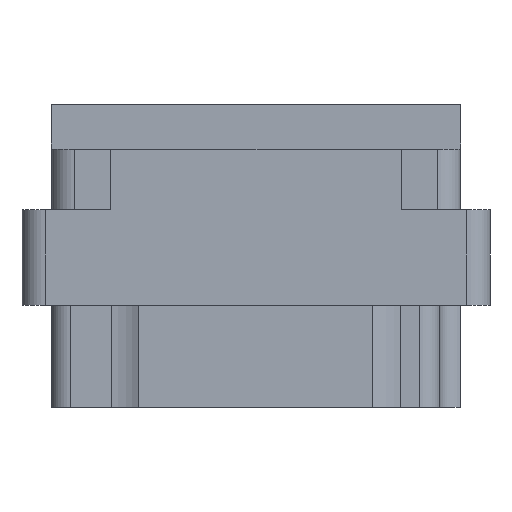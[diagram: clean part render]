
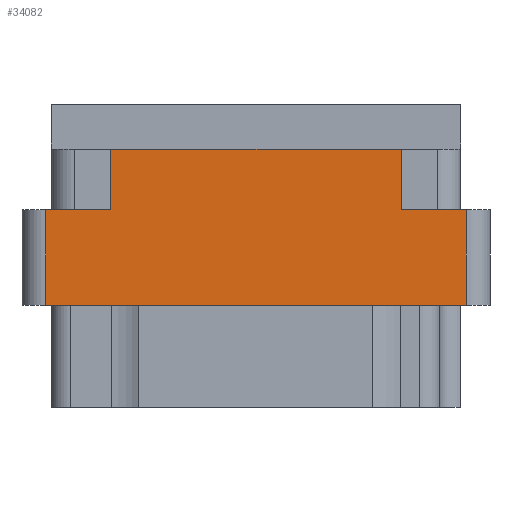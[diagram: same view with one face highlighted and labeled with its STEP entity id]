
A CAD part, left-side view. The second image highlights one B-rep face of the part: STEP entity #34082.
In plain terms, the highlighted planar face has unit normal (-1, 0, 0).
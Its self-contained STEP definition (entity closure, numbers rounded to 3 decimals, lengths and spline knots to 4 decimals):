
#12 = CARTESIAN_POINT ( 'NONE',  ( -1.359, 0.617, -0.117 ) ) ;
#473 = VECTOR ( 'NONE', #33977, 39.3701 ) ;
#823 = VERTEX_POINT ( 'NONE', #48554 ) ;
#3476 = EDGE_CURVE ( 'NONE', #823, #56466, #4564, .T. ) ;
#3737 = CARTESIAN_POINT ( 'NONE',  ( -1.359, -0.3825, -0.277 ) ) ;
#4472 = CARTESIAN_POINT ( 'NONE',  ( -1.359, -0.3825, -0.117 ) ) ;
#4564 = LINE ( 'NONE', #55939, #473 ) ;
#5445 = VERTEX_POINT ( 'NONE', #45463 ) ;
#5642 = VERTEX_POINT ( 'NONE', #42252 ) ;
#6634 = DIRECTION ( 'NONE',  ( 0., 0., 1. ) ) ;
#6751 = LINE ( 'NONE', #41311, #39908 ) ;
#8000 = LINE ( 'NONE', #8088, #42814 ) ;
#8088 = CARTESIAN_POINT ( 'NONE',  ( -1.359, 0.555, -0.798 ) ) ;
#11382 = VERTEX_POINT ( 'NONE', #18993 ) ;
#11663 = LINE ( 'NONE', #57375, #38190 ) ;
#14335 = LINE ( 'NONE', #16645, #18534 ) ;
#14770 = ORIENTED_EDGE ( 'NONE', *, *, #55445, .F. ) ;
#15271 = DIRECTION ( 'NONE',  ( 0., -1., 0. ) ) ;
#15533 = EDGE_CURVE ( 'NONE', #11382, #64321, #14335, .T. ) ;
#16645 = CARTESIAN_POINT ( 'NONE',  ( -1.359, 0., -0.529 ) ) ;
#18534 = VECTOR ( 'NONE', #21676, 39.3701 ) ;
#18692 = VERTEX_POINT ( 'NONE', #60002 ) ;
#18993 = CARTESIAN_POINT ( 'NONE',  ( -1.359, -0.555, -0.529 ) ) ;
#19235 = ORIENTED_EDGE ( 'NONE', *, *, #15533, .F. ) ;
#19709 = LINE ( 'NONE', #12, #23008 ) ;
#20293 = FACE_OUTER_BOUND ( 'NONE', #48943, .T. ) ;
#20583 = DIRECTION ( 'NONE',  ( 0., 0., 1. ) ) ;
#21238 = CARTESIAN_POINT ( 'NONE',  ( -1.359, 0.3825, -0.277 ) ) ;
#21350 = ORIENTED_EDGE ( 'NONE', *, *, #66584, .T. ) ;
#21676 = DIRECTION ( 'NONE',  ( 0., 1., 0. ) ) ;
#22832 = PLANE ( 'NONE',  #50138 ) ;
#23008 = VECTOR ( 'NONE', #15271, 39.3701 ) ;
#24571 = DIRECTION ( 'NONE',  ( 0., 0., 1. ) ) ;
#28092 = VECTOR ( 'NONE', #39802, 39.3701 ) ;
#28145 = EDGE_CURVE ( 'NONE', #11382, #5445, #11663, .T. ) ;
#29629 = CARTESIAN_POINT ( 'NONE',  ( -1.359, 0.3825, -0.277 ) ) ;
#30195 = ORIENTED_EDGE ( 'NONE', *, *, #28145, .T. ) ;
#33558 = EDGE_CURVE ( 'NONE', #18692, #34763, #34463, .T. ) ;
#33977 = DIRECTION ( 'NONE',  ( 0., -1., 0. ) ) ;
#34082 = ADVANCED_FACE ( 'NONE', ( #20293 ), #22832, .T. ) ;
#34463 = LINE ( 'NONE', #3737, #60959 ) ;
#34763 = VERTEX_POINT ( 'NONE', #4472 ) ;
#38190 = VECTOR ( 'NONE', #20583, 39.3701 ) ;
#39802 = DIRECTION ( 'NONE',  ( 0., 0., 1. ) ) ;
#39908 = VECTOR ( 'NONE', #61441, 39.3701 ) ;
#41311 = CARTESIAN_POINT ( 'NONE',  ( -1.359, 0., -0.277 ) ) ;
#42252 = CARTESIAN_POINT ( 'NONE',  ( -1.359, 0.3825, -0.117 ) ) ;
#42814 = VECTOR ( 'NONE', #45092, 39.3701 ) ;
#45092 = DIRECTION ( 'NONE',  ( 0., 0., -1. ) ) ;
#45463 = CARTESIAN_POINT ( 'NONE',  ( -1.359, -0.555, -0.277 ) ) ;
#47794 = CARTESIAN_POINT ( 'NONE',  ( -1.359, 0.555, -0.529 ) ) ;
#48554 = CARTESIAN_POINT ( 'NONE',  ( -1.359, 0.555, -0.277 ) ) ;
#48716 = EDGE_CURVE ( 'NONE', #56466, #5642, #64538, .T. ) ;
#48943 = EDGE_LOOP ( 'NONE', ( #52334, #21350, #19235, #30195, #14770, #51629, #66566, #64814 ) ) ;
#50138 = AXIS2_PLACEMENT_3D ( 'NONE', #64931, #65377, #6634 ) ;
#51629 = ORIENTED_EDGE ( 'NONE', *, *, #33558, .T. ) ;
#52264 = EDGE_CURVE ( 'NONE', #5642, #34763, #19709, .T. ) ;
#52334 = ORIENTED_EDGE ( 'NONE', *, *, #3476, .F. ) ;
#55445 = EDGE_CURVE ( 'NONE', #18692, #5445, #6751, .T. ) ;
#55939 = CARTESIAN_POINT ( 'NONE',  ( -1.359, 0., -0.277 ) ) ;
#56466 = VERTEX_POINT ( 'NONE', #21238 ) ;
#57375 = CARTESIAN_POINT ( 'NONE',  ( -1.359, -0.555, -0.798 ) ) ;
#60002 = CARTESIAN_POINT ( 'NONE',  ( -1.359, -0.3825, -0.277 ) ) ;
#60959 = VECTOR ( 'NONE', #24571, 39.3701 ) ;
#61441 = DIRECTION ( 'NONE',  ( 0., -1., 0. ) ) ;
#64321 = VERTEX_POINT ( 'NONE', #47794 ) ;
#64538 = LINE ( 'NONE', #29629, #28092 ) ;
#64814 = ORIENTED_EDGE ( 'NONE', *, *, #48716, .F. ) ;
#64931 = CARTESIAN_POINT ( 'NONE',  ( -1.359, -0.617, -0.798 ) ) ;
#65377 = DIRECTION ( 'NONE',  ( -1., 0., 0. ) ) ;
#66566 = ORIENTED_EDGE ( 'NONE', *, *, #52264, .F. ) ;
#66584 = EDGE_CURVE ( 'NONE', #823, #64321, #8000, .T. ) ;
